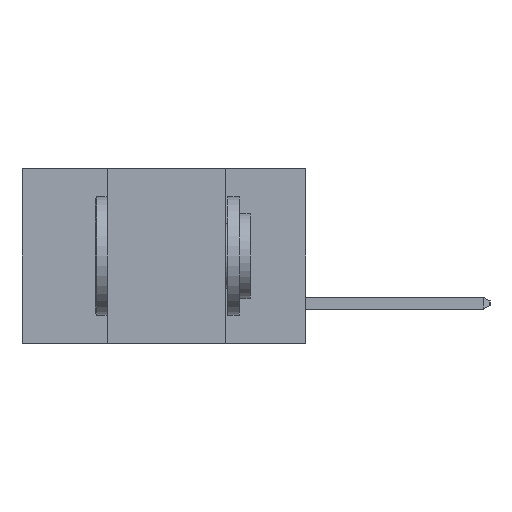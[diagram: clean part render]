
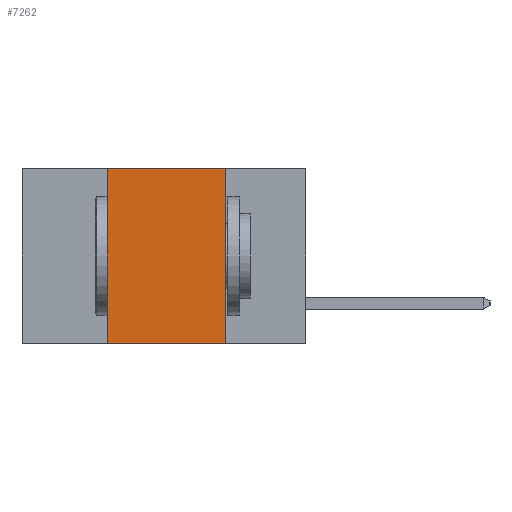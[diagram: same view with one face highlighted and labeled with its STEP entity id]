
A CAD part, left-side view. The second image highlights one B-rep face of the part: STEP entity #7262.
In plain terms, the highlighted planar face has unit normal (-1, 0, 0).
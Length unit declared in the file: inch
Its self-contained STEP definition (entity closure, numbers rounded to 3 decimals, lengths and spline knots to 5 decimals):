
#529 = CARTESIAN_POINT ( 'NONE',  ( 0., 0.42, 0. ) ) ;
#1459 = FACE_OUTER_BOUND ( 'NONE', #6844, .T. ) ;
#4095 = LINE ( 'NONE', #15357, #14550 ) ;
#4450 = DIRECTION ( 'NONE',  ( 0., 0., -1. ) ) ;
#5207 = VERTEX_POINT ( 'NONE', #10908 ) ;
#5815 = CARTESIAN_POINT ( 'NONE',  ( 0., 0.42, -0.37 ) ) ;
#5980 = EDGE_CURVE ( 'NONE', #17424, #5207, #12429, .T. ) ;
#6699 = CARTESIAN_POINT ( 'NONE',  ( 0., 0.6, 0. ) ) ;
#6740 = DIRECTION ( 'NONE',  ( 1., 0., 0. ) ) ;
#6809 = ORIENTED_EDGE ( 'NONE', *, *, #8423, .F. ) ;
#6844 = EDGE_LOOP ( 'NONE', ( #13576, #6809, #15537, #11703 ) ) ;
#6923 = AXIS2_PLACEMENT_3D ( 'NONE', #14874, #6740, #16257 ) ;
#7169 = DIRECTION ( 'NONE',  ( 0., 0., 1. ) ) ;
#7262 = ADVANCED_FACE ( 'NONE', ( #1459 ), #12135, .F. ) ;
#8093 = DIRECTION ( 'NONE',  ( 0., -1., 0. ) ) ;
#8423 = EDGE_CURVE ( 'NONE', #17795, #8598, #8916, .T. ) ;
#8491 = VECTOR ( 'NONE', #8093, 39.37008 ) ;
#8598 = VERTEX_POINT ( 'NONE', #12454 ) ;
#8842 = DIRECTION ( 'NONE',  ( 0., -1., 0. ) ) ;
#8916 = LINE ( 'NONE', #6699, #8491 ) ;
#9955 = VECTOR ( 'NONE', #7169, 39.37008 ) ;
#10370 = LINE ( 'NONE', #5815, #9955 ) ;
#10600 = EDGE_CURVE ( 'NONE', #17424, #17795, #10370, .T. ) ;
#10908 = CARTESIAN_POINT ( 'NONE',  ( 0., 0.17, -0.37 ) ) ;
#11703 = ORIENTED_EDGE ( 'NONE', *, *, #5980, .T. ) ;
#12135 = PLANE ( 'NONE',  #6923 ) ;
#12429 = LINE ( 'NONE', #15595, #15196 ) ;
#12454 = CARTESIAN_POINT ( 'NONE',  ( 0., 0.17, 0. ) ) ;
#13576 = ORIENTED_EDGE ( 'NONE', *, *, #15128, .F. ) ;
#14550 = VECTOR ( 'NONE', #4450, 39.37008 ) ;
#14720 = CARTESIAN_POINT ( 'NONE',  ( 0., 0.42, -0.37 ) ) ;
#14874 = CARTESIAN_POINT ( 'NONE',  ( 0., 0.6, 0. ) ) ;
#15128 = EDGE_CURVE ( 'NONE', #8598, #5207, #4095, .T. ) ;
#15196 = VECTOR ( 'NONE', #8842, 39.37008 ) ;
#15357 = CARTESIAN_POINT ( 'NONE',  ( 0., 0.17, -0.37 ) ) ;
#15537 = ORIENTED_EDGE ( 'NONE', *, *, #10600, .F. ) ;
#15595 = CARTESIAN_POINT ( 'NONE',  ( 0., 0.6, -0.37 ) ) ;
#16257 = DIRECTION ( 'NONE',  ( 0., 0., -1. ) ) ;
#17424 = VERTEX_POINT ( 'NONE', #14720 ) ;
#17795 = VERTEX_POINT ( 'NONE', #529 ) ;
